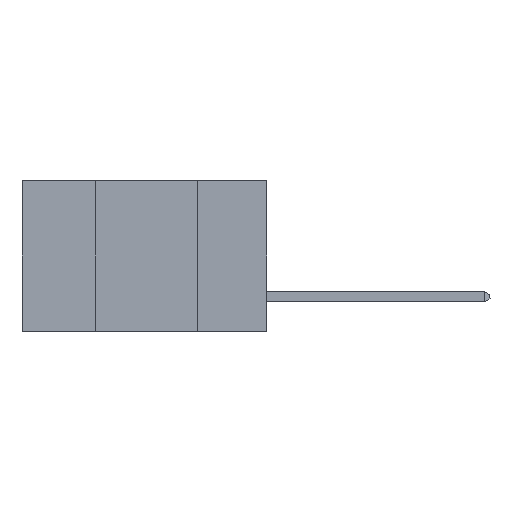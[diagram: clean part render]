
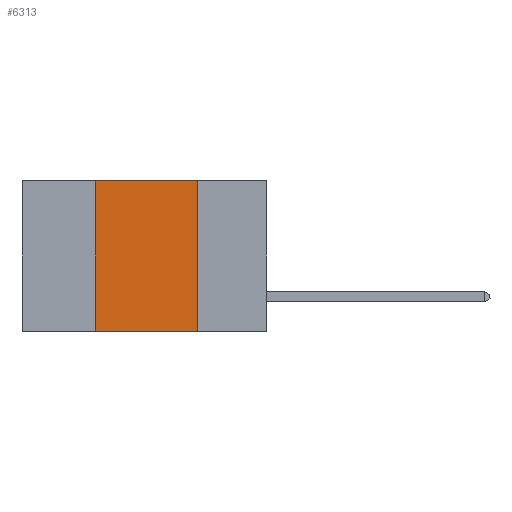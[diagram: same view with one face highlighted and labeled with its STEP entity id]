
A CAD part, left-side view. The second image highlights one B-rep face of the part: STEP entity #6313.
In plain terms, the highlighted planar face has unit normal (-1, 0, 0).
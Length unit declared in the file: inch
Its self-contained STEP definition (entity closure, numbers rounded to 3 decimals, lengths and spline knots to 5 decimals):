
#169 = LINE ( 'NONE', #3520, #4318 ) ;
#358 = EDGE_CURVE ( 'NONE', #7433, #5503, #10022, .T. ) ;
#962 = CARTESIAN_POINT ( 'NONE',  ( 0., 0.6, 0. ) ) ;
#2158 = DIRECTION ( 'NONE',  ( 1., 0., 0. ) ) ;
#2322 = ORIENTED_EDGE ( 'NONE', *, *, #7282, .T. ) ;
#2492 = DIRECTION ( 'NONE',  ( 0., -1., 0. ) ) ;
#2553 = LINE ( 'NONE', #962, #8340 ) ;
#2902 = CARTESIAN_POINT ( 'NONE',  ( 0., 0.17, 0. ) ) ;
#3329 = VERTEX_POINT ( 'NONE', #5716 ) ;
#3422 = CARTESIAN_POINT ( 'NONE',  ( 0., 0.17, 0. ) ) ;
#3520 = CARTESIAN_POINT ( 'NONE',  ( 0., 0.6, -0.37 ) ) ;
#3688 = FACE_OUTER_BOUND ( 'NONE', #4292, .T. ) ;
#3798 = ORIENTED_EDGE ( 'NONE', *, *, #9546, .F. ) ;
#3966 = ORIENTED_EDGE ( 'NONE', *, *, #6045, .F. ) ;
#4018 = ORIENTED_EDGE ( 'NONE', *, *, #358, .F. ) ;
#4193 = CARTESIAN_POINT ( 'NONE',  ( 0., 0.17, -0.37 ) ) ;
#4292 = EDGE_LOOP ( 'NONE', ( #4018, #3966, #3798, #2322 ) ) ;
#4318 = VECTOR ( 'NONE', #7480, 39.37008 ) ;
#4407 = VECTOR ( 'NONE', #6626, 39.37008 ) ;
#4630 = PLANE ( 'NONE',  #6228 ) ;
#5344 = DIRECTION ( 'NONE',  ( 0., 0., -1. ) ) ;
#5503 = VERTEX_POINT ( 'NONE', #4193 ) ;
#5716 = CARTESIAN_POINT ( 'NONE',  ( 0., 0.42, 0. ) ) ;
#5832 = CARTESIAN_POINT ( 'NONE',  ( 0., 0.42, 0. ) ) ;
#6045 = EDGE_CURVE ( 'NONE', #3329, #7433, #2553, .T. ) ;
#6228 = AXIS2_PLACEMENT_3D ( 'NONE', #7764, #2158, #10119 ) ;
#6313 = ADVANCED_FACE ( 'NONE', ( #3688 ), #4630, .F. ) ;
#6393 = VECTOR ( 'NONE', #5344, 39.37008 ) ;
#6626 = DIRECTION ( 'NONE',  ( 0., 0., 1. ) ) ;
#7257 = VERTEX_POINT ( 'NONE', #8828 ) ;
#7282 = EDGE_CURVE ( 'NONE', #7257, #5503, #169, .T. ) ;
#7433 = VERTEX_POINT ( 'NONE', #2902 ) ;
#7480 = DIRECTION ( 'NONE',  ( 0., -1., 0. ) ) ;
#7764 = CARTESIAN_POINT ( 'NONE',  ( 0., 0.6, 0. ) ) ;
#8340 = VECTOR ( 'NONE', #2492, 39.37008 ) ;
#8397 = LINE ( 'NONE', #5832, #4407 ) ;
#8828 = CARTESIAN_POINT ( 'NONE',  ( 0., 0.42, -0.37 ) ) ;
#9546 = EDGE_CURVE ( 'NONE', #7257, #3329, #8397, .T. ) ;
#10022 = LINE ( 'NONE', #3422, #6393 ) ;
#10119 = DIRECTION ( 'NONE',  ( 0., 0., -1. ) ) ;
